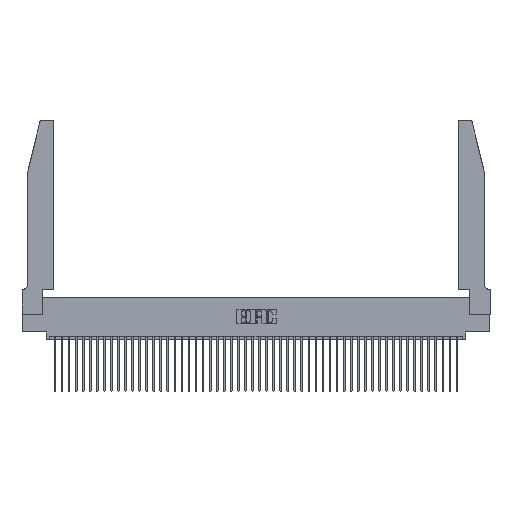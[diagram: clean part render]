
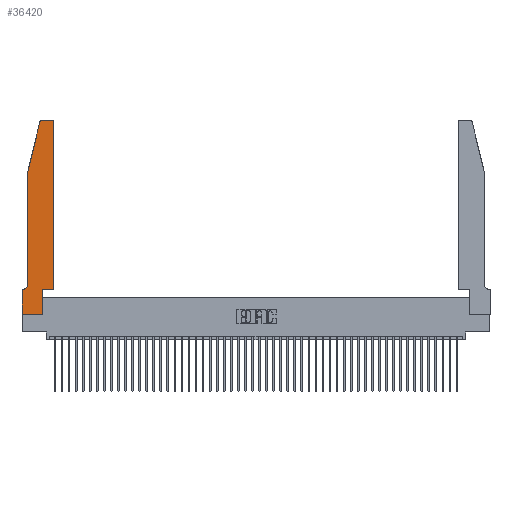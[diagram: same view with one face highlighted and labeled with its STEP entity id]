
A CAD part, top view. The second image highlights one B-rep face of the part: STEP entity #36420.
In plain terms, the highlighted planar face has unit normal (0, 0, 1).
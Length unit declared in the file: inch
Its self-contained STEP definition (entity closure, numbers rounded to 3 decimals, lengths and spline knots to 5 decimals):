
#1596 = VERTEX_POINT ( 'NONE', #32794 ) ;
#2361 = EDGE_CURVE ( 'NONE', #21235, #7903, #45707, .T. ) ;
#3081 = CARTESIAN_POINT ( 'NONE',  ( 0.4205, 2.72, 0.37 ) ) ;
#3306 = EDGE_CURVE ( 'NONE', #8084, #35778, #33401, .T. ) ;
#3407 = LINE ( 'NONE', #31838, #32009 ) ;
#3524 = LINE ( 'NONE', #35996, #11687 ) ;
#4677 = ORIENTED_EDGE ( 'NONE', *, *, #25312, .T. ) ;
#4831 = CARTESIAN_POINT ( 'NONE',  ( 0.4505, 0.35, 0.37 ) ) ;
#5737 = EDGE_CURVE ( 'NONE', #28557, #38712, #30521, .T. ) ;
#5960 = VECTOR ( 'NONE', #15675, 39.37008 ) ;
#6284 = DIRECTION ( 'NONE',  ( -1., 0., 0. ) ) ;
#6735 = AXIS2_PLACEMENT_3D ( 'NONE', #32815, #10477, #14237 ) ;
#6824 = CARTESIAN_POINT ( 'NONE',  ( 0., 0., 0.37 ) ) ;
#7556 = CIRCLE ( 'NONE', #6735, 0.07 ) ;
#7609 = CARTESIAN_POINT ( 'NONE',  ( 0.2605, 2.75, 0.37 ) ) ;
#7903 = VERTEX_POINT ( 'NONE', #29796 ) ;
#8045 = CARTESIAN_POINT ( 'NONE',  ( 0.0755, 2., 0.37 ) ) ;
#8084 = VERTEX_POINT ( 'NONE', #41642 ) ;
#8240 = VECTOR ( 'NONE', #42631, 39.37008 ) ;
#8267 = FACE_OUTER_BOUND ( 'NONE', #47355, .T. ) ;
#8817 = EDGE_CURVE ( 'NONE', #1596, #38634, #3407, .T. ) ;
#9782 = EDGE_CURVE ( 'NONE', #7903, #8084, #20838, .T. ) ;
#9795 = EDGE_CURVE ( 'NONE', #19399, #21235, #14437, .T. ) ;
#9903 = CARTESIAN_POINT ( 'NONE',  ( 0.284, 2.72, 0.37 ) ) ;
#10477 = DIRECTION ( 'NONE',  ( 0., 0., -1. ) ) ;
#11687 = VECTOR ( 'NONE', #29128, 39.37008 ) ;
#12806 = EDGE_CURVE ( 'NONE', #32875, #1596, #41716, .T. ) ;
#13138 = CARTESIAN_POINT ( 'NONE',  ( 0.25487, 2.72718, 0.37 ) ) ;
#13669 = DIRECTION ( 'NONE',  ( 0., 0., 1. ) ) ;
#14237 = DIRECTION ( 'NONE',  ( -1., 0., 0. ) ) ;
#14437 = LINE ( 'NONE', #33691, #17346 ) ;
#15675 = DIRECTION ( 'NONE',  ( 0., 1., 0. ) ) ;
#17083 = AXIS2_PLACEMENT_3D ( 'NONE', #35550, #35862, #28073 ) ;
#17346 = VECTOR ( 'NONE', #19023, 39.37008 ) ;
#17348 = DIRECTION ( 'NONE',  ( 0., -1., 0. ) ) ;
#17388 = CARTESIAN_POINT ( 'NONE',  ( 0.0055, 0.35, 0.37 ) ) ;
#17861 = VECTOR ( 'NONE', #19914, 39.37008 ) ;
#17984 = ORIENTED_EDGE ( 'NONE', *, *, #3306, .T. ) ;
#19023 = DIRECTION ( 'NONE',  ( 0., 1., 0. ) ) ;
#19399 = VERTEX_POINT ( 'NONE', #46774 ) ;
#19499 = VERTEX_POINT ( 'NONE', #26147 ) ;
#19914 = DIRECTION ( 'NONE',  ( 0., -1., 0. ) ) ;
#20510 = LINE ( 'NONE', #4831, #29248 ) ;
#20678 = EDGE_CURVE ( 'NONE', #35778, #21460, #3524, .T. ) ;
#20838 = LINE ( 'NONE', #7609, #34237 ) ;
#21170 = ORIENTED_EDGE ( 'NONE', *, *, #12806, .T. ) ;
#21235 = VERTEX_POINT ( 'NONE', #43081 ) ;
#21460 = VERTEX_POINT ( 'NONE', #8045 ) ;
#23322 = CARTESIAN_POINT ( 'NONE',  ( 0.0755, 2., 0.37 ) ) ;
#24515 = CARTESIAN_POINT ( 'NONE',  ( 0.2865, 0., 0.37 ) ) ;
#24630 = PLANE ( 'NONE',  #17083 ) ;
#25312 = EDGE_CURVE ( 'NONE', #38712, #19399, #20510, .T. ) ;
#25885 = EDGE_CURVE ( 'NONE', #38634, #28557, #33869, .T. ) ;
#26147 = CARTESIAN_POINT ( 'NONE',  ( 0.0755, 0.42, 0.37 ) ) ;
#27052 = CARTESIAN_POINT ( 'NONE',  ( 0.2865, 0.35, 0.37 ) ) ;
#27806 = DIRECTION ( 'NONE',  ( 0., 0., 1. ) ) ;
#27997 = CARTESIAN_POINT ( 'NONE',  ( 0., 0., 0.37 ) ) ;
#28073 = DIRECTION ( 'NONE',  ( 1., 0., 0. ) ) ;
#28557 = VERTEX_POINT ( 'NONE', #24515 ) ;
#28880 = VECTOR ( 'NONE', #6284, 39.37008 ) ;
#28909 = EDGE_CURVE ( 'NONE', #21460, #19499, #37659, .T. ) ;
#29128 = DIRECTION ( 'NONE',  ( -0.239, -0.971, 0. ) ) ;
#29248 = VECTOR ( 'NONE', #31104, 39.37008 ) ;
#29355 = CARTESIAN_POINT ( 'NONE',  ( 0.2865, 0.35, 0.37 ) ) ;
#29443 = ORIENTED_EDGE ( 'NONE', *, *, #8817, .T. ) ;
#29796 = CARTESIAN_POINT ( 'NONE',  ( 0.4205, 2.75, 0.37 ) ) ;
#30178 = ORIENTED_EDGE ( 'NONE', *, *, #9782, .T. ) ;
#30521 = LINE ( 'NONE', #27052, #5960 ) ;
#31104 = DIRECTION ( 'NONE',  ( 1., 0., 0. ) ) ;
#31838 = CARTESIAN_POINT ( 'NONE',  ( 0., 0., 0.37 ) ) ;
#32009 = VECTOR ( 'NONE', #17348, 39.37008 ) ;
#32794 = CARTESIAN_POINT ( 'NONE',  ( 0., 0.35, 0.37 ) ) ;
#32815 = CARTESIAN_POINT ( 'NONE',  ( 0.0055, 0.42, 0.37 ) ) ;
#32875 = VERTEX_POINT ( 'NONE', #17388 ) ;
#33401 = CIRCLE ( 'NONE', #43379, 0.03 ) ;
#33535 = ORIENTED_EDGE ( 'NONE', *, *, #28909, .T. ) ;
#33691 = CARTESIAN_POINT ( 'NONE',  ( 0.4505, 0.35, 0.37 ) ) ;
#33869 = LINE ( 'NONE', #27997, #8240 ) ;
#34237 = VECTOR ( 'NONE', #41000, 39.37008 ) ;
#35550 = CARTESIAN_POINT ( 'NONE',  ( 0., 0.35, 0.37 ) ) ;
#35778 = VERTEX_POINT ( 'NONE', #13138 ) ;
#35862 = DIRECTION ( 'NONE',  ( 0., 0., 1. ) ) ;
#35996 = CARTESIAN_POINT ( 'NONE',  ( 0.0755, 2., 0.37 ) ) ;
#36420 = ADVANCED_FACE ( 'NONE', ( #8267 ), #24630, .T. ) ;
#37659 = LINE ( 'NONE', #23322, #17861 ) ;
#38038 = EDGE_CURVE ( 'NONE', #19499, #32875, #7556, .T. ) ;
#38634 = VERTEX_POINT ( 'NONE', #6824 ) ;
#38712 = VERTEX_POINT ( 'NONE', #29355 ) ;
#38891 = ORIENTED_EDGE ( 'NONE', *, *, #25885, .T. ) ;
#39597 = AXIS2_PLACEMENT_3D ( 'NONE', #3081, #27806, #39942 ) ;
#39942 = DIRECTION ( 'NONE',  ( 1., 0., 0. ) ) ;
#41000 = DIRECTION ( 'NONE',  ( -1., 0., 0. ) ) ;
#41642 = CARTESIAN_POINT ( 'NONE',  ( 0.284, 2.75, 0.37 ) ) ;
#41716 = LINE ( 'NONE', #47501, #28880 ) ;
#42368 = ORIENTED_EDGE ( 'NONE', *, *, #20678, .T. ) ;
#42465 = ORIENTED_EDGE ( 'NONE', *, *, #2361, .T. ) ;
#42631 = DIRECTION ( 'NONE',  ( 1., 0., 0. ) ) ;
#43063 = ORIENTED_EDGE ( 'NONE', *, *, #38038, .T. ) ;
#43081 = CARTESIAN_POINT ( 'NONE',  ( 0.4505, 2.72, 0.37 ) ) ;
#43379 = AXIS2_PLACEMENT_3D ( 'NONE', #9903, #13669, #47195 ) ;
#45707 = CIRCLE ( 'NONE', #39597, 0.03 ) ;
#46774 = CARTESIAN_POINT ( 'NONE',  ( 0.4505, 0.35, 0.37 ) ) ;
#47195 = DIRECTION ( 'NONE',  ( 1., 0., 0. ) ) ;
#47355 = EDGE_LOOP ( 'NONE', ( #30178, #17984, #42368, #33535, #43063, #21170, #29443, #38891, #47987, #4677, #47873, #42465 ) ) ;
#47501 = CARTESIAN_POINT ( 'NONE',  ( 0.0755, 0.35, 0.37 ) ) ;
#47873 = ORIENTED_EDGE ( 'NONE', *, *, #9795, .T. ) ;
#47987 = ORIENTED_EDGE ( 'NONE', *, *, #5737, .T. ) ;
